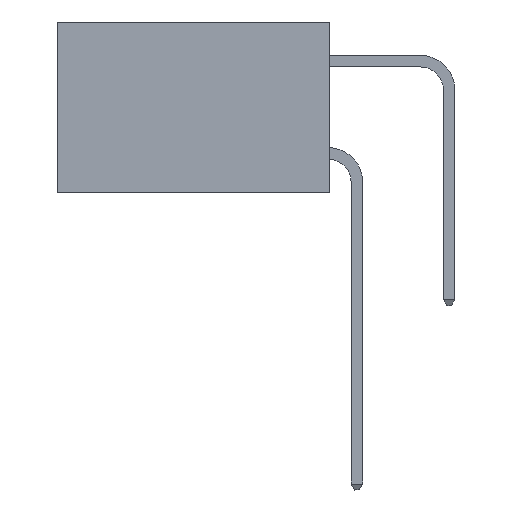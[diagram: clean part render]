
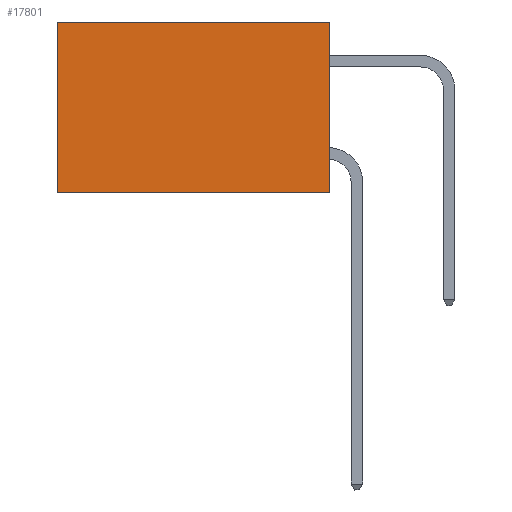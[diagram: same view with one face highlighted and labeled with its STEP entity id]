
A CAD part, left-side view. The second image highlights one B-rep face of the part: STEP entity #17801.
In plain terms, the highlighted planar face has unit normal (-1, 0, 0).
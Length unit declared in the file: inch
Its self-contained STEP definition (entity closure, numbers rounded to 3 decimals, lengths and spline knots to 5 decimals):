
#231 = VECTOR ( 'NONE', #16766, 39.37008 ) ;
#243 = CARTESIAN_POINT ( 'NONE',  ( 0.277, 0., -0.37 ) ) ;
#629 = VERTEX_POINT ( 'NONE', #6268 ) ;
#822 = VECTOR ( 'NONE', #18122, 39.37008 ) ;
#1610 = EDGE_CURVE ( 'NONE', #17468, #19513, #20528, .T. ) ;
#2240 = EDGE_CURVE ( 'NONE', #15086, #17468, #13295, .T. ) ;
#2402 = ORIENTED_EDGE ( 'NONE', *, *, #2240, .F. ) ;
#2934 = CARTESIAN_POINT ( 'NONE',  ( 0.277, 0., -0.37 ) ) ;
#5262 = PLANE ( 'NONE',  #9912 ) ;
#6268 = CARTESIAN_POINT ( 'NONE',  ( 0.277, 0.59, 0. ) ) ;
#6599 = VECTOR ( 'NONE', #18529, 39.37008 ) ;
#6912 = DIRECTION ( 'NONE',  ( 1., 0., 0. ) ) ;
#8465 = DIRECTION ( 'NONE',  ( 0., 1., 0. ) ) ;
#9224 = CARTESIAN_POINT ( 'NONE',  ( 0.277, 0.59, -0.37 ) ) ;
#9311 = CARTESIAN_POINT ( 'NONE',  ( 0.277, 0., 0. ) ) ;
#9912 = AXIS2_PLACEMENT_3D ( 'NONE', #243, #6912, #17958 ) ;
#10326 = VECTOR ( 'NONE', #8465, 39.37008 ) ;
#10452 = FACE_OUTER_BOUND ( 'NONE', #15202, .T. ) ;
#11013 = LINE ( 'NONE', #9224, #6599 ) ;
#12006 = CARTESIAN_POINT ( 'NONE',  ( 0.277, 0., -0.37 ) ) ;
#12964 = EDGE_CURVE ( 'NONE', #15086, #629, #18055, .T. ) ;
#13295 = LINE ( 'NONE', #12006, #231 ) ;
#13842 = ORIENTED_EDGE ( 'NONE', *, *, #1610, .F. ) ;
#15086 = VERTEX_POINT ( 'NONE', #9311 ) ;
#15202 = EDGE_LOOP ( 'NONE', ( #17457, #13842, #2402, #15651 ) ) ;
#15651 = ORIENTED_EDGE ( 'NONE', *, *, #12964, .T. ) ;
#16348 = EDGE_CURVE ( 'NONE', #629, #19513, #11013, .T. ) ;
#16766 = DIRECTION ( 'NONE',  ( 0., 0., -1. ) ) ;
#17457 = ORIENTED_EDGE ( 'NONE', *, *, #16348, .T. ) ;
#17468 = VERTEX_POINT ( 'NONE', #2934 ) ;
#17801 = ADVANCED_FACE ( 'NONE', ( #10452 ), #5262, .F. ) ;
#17868 = CARTESIAN_POINT ( 'NONE',  ( 0.277, 0., 0. ) ) ;
#17958 = DIRECTION ( 'NONE',  ( 0., 0., -1. ) ) ;
#18049 = CARTESIAN_POINT ( 'NONE',  ( 0.277, 0.59, -0.37 ) ) ;
#18055 = LINE ( 'NONE', #17868, #10326 ) ;
#18122 = DIRECTION ( 'NONE',  ( 0., 1., 0. ) ) ;
#18529 = DIRECTION ( 'NONE',  ( 0., 0., -1. ) ) ;
#18547 = CARTESIAN_POINT ( 'NONE',  ( 0.277, 0., -0.37 ) ) ;
#19513 = VERTEX_POINT ( 'NONE', #18049 ) ;
#20528 = LINE ( 'NONE', #18547, #822 ) ;
